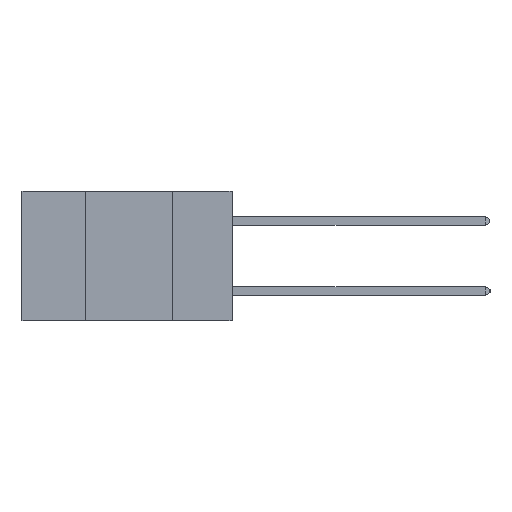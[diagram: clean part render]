
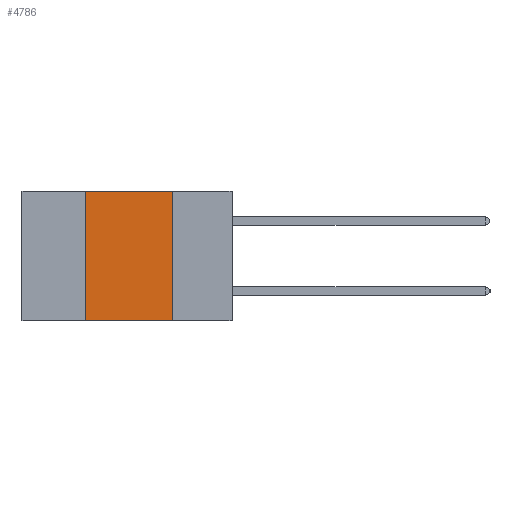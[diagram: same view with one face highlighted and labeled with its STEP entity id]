
A CAD part, left-side view. The second image highlights one B-rep face of the part: STEP entity #4786.
In plain terms, the highlighted planar face has unit normal (-1, 0, 0).
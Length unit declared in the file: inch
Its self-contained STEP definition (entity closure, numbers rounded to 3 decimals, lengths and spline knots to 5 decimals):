
#360 = CARTESIAN_POINT ( 'NONE',  ( 0., 0.17, 0. ) ) ;
#534 = DIRECTION ( 'NONE',  ( 0., -1., 0. ) ) ;
#699 = FACE_OUTER_BOUND ( 'NONE', #1146, .T. ) ;
#1146 = EDGE_LOOP ( 'NONE', ( #17241, #5066, #6677, #11632 ) ) ;
#1661 = VECTOR ( 'NONE', #12718, 39.37008 ) ;
#2541 = LINE ( 'NONE', #3349, #18387 ) ;
#2967 = VECTOR ( 'NONE', #534, 39.37008 ) ;
#3349 = CARTESIAN_POINT ( 'NONE',  ( 0., 0.17, 0. ) ) ;
#3661 = DIRECTION ( 'NONE',  ( 1., 0., 0. ) ) ;
#3725 = DIRECTION ( 'NONE',  ( 0., 0., 1. ) ) ;
#3994 = CARTESIAN_POINT ( 'NONE',  ( 0., 0.42, 0. ) ) ;
#4038 = EDGE_CURVE ( 'NONE', #9742, #12801, #18199, .T. ) ;
#4786 = ADVANCED_FACE ( 'NONE', ( #699 ), #6512, .F. ) ;
#5066 = ORIENTED_EDGE ( 'NONE', *, *, #15695, .F. ) ;
#5584 = LINE ( 'NONE', #15618, #1661 ) ;
#6031 = VERTEX_POINT ( 'NONE', #360 ) ;
#6512 = PLANE ( 'NONE',  #12524 ) ;
#6677 = ORIENTED_EDGE ( 'NONE', *, *, #4038, .F. ) ;
#7481 = CARTESIAN_POINT ( 'NONE',  ( 0., 0.42, 0. ) ) ;
#9742 = VERTEX_POINT ( 'NONE', #17148 ) ;
#11632 = ORIENTED_EDGE ( 'NONE', *, *, #16932, .T. ) ;
#11916 = CARTESIAN_POINT ( 'NONE',  ( 0., 0.17, -0.37 ) ) ;
#12524 = AXIS2_PLACEMENT_3D ( 'NONE', #12693, #3661, #14194 ) ;
#12553 = CARTESIAN_POINT ( 'NONE',  ( 0., 0.6, -0.37 ) ) ;
#12693 = CARTESIAN_POINT ( 'NONE',  ( 0., 0.6, 0. ) ) ;
#12718 = DIRECTION ( 'NONE',  ( 0., -1., 0. ) ) ;
#12801 = VERTEX_POINT ( 'NONE', #7481 ) ;
#13877 = DIRECTION ( 'NONE',  ( 0., 0., -1. ) ) ;
#14194 = DIRECTION ( 'NONE',  ( 0., 0., -1. ) ) ;
#14965 = LINE ( 'NONE', #12553, #2967 ) ;
#15403 = VERTEX_POINT ( 'NONE', #11916 ) ;
#15618 = CARTESIAN_POINT ( 'NONE',  ( 0., 0.6, 0. ) ) ;
#15695 = EDGE_CURVE ( 'NONE', #12801, #6031, #5584, .T. ) ;
#16092 = EDGE_CURVE ( 'NONE', #6031, #15403, #2541, .T. ) ;
#16932 = EDGE_CURVE ( 'NONE', #9742, #15403, #14965, .T. ) ;
#17148 = CARTESIAN_POINT ( 'NONE',  ( 0., 0.42, -0.37 ) ) ;
#17241 = ORIENTED_EDGE ( 'NONE', *, *, #16092, .F. ) ;
#18199 = LINE ( 'NONE', #3994, #19087 ) ;
#18387 = VECTOR ( 'NONE', #13877, 39.37008 ) ;
#19087 = VECTOR ( 'NONE', #3725, 39.37008 ) ;
